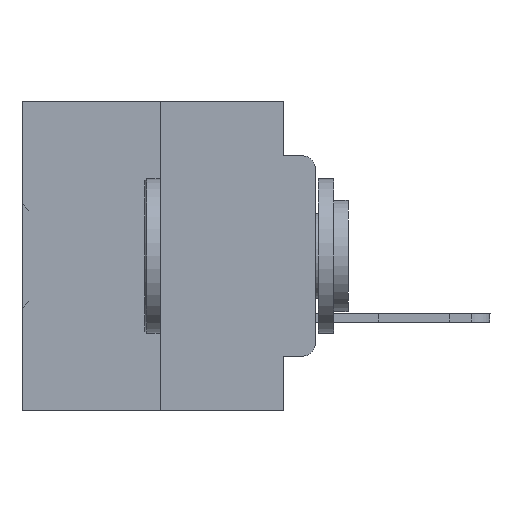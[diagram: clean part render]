
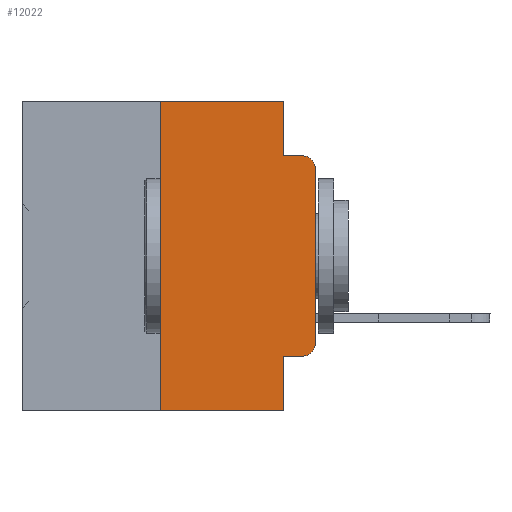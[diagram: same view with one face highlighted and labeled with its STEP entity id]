
A CAD part, left-side view. The second image highlights one B-rep face of the part: STEP entity #12022.
In plain terms, the highlighted planar face has unit normal (-1, 0, 0).
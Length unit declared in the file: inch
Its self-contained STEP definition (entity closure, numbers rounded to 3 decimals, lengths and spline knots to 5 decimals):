
#242 = CARTESIAN_POINT ( 'NONE',  ( 0., 0.051, -0.5 ) ) ;
#499 = VERTEX_POINT ( 'NONE', #16142 ) ;
#1113 = VERTEX_POINT ( 'NONE', #6329 ) ;
#1200 = CARTESIAN_POINT ( 'NONE',  ( 0., 0., 0. ) ) ;
#1485 = ORIENTED_EDGE ( 'NONE', *, *, #6885, .T. ) ;
#2350 = EDGE_LOOP ( 'NONE', ( #1485, #3402, #27702, #34656, #17338, #6366, #14215, #23502, #6802, #17267 ) ) ;
#2783 = CARTESIAN_POINT ( 'NONE',  ( 0., 0.051, 0. ) ) ;
#3402 = ORIENTED_EDGE ( 'NONE', *, *, #23648, .T. ) ;
#3685 = EDGE_CURVE ( 'NONE', #499, #12463, #12666, .T. ) ;
#3968 = AXIS2_PLACEMENT_3D ( 'NONE', #9391, #18183, #12584 ) ;
#4217 = CARTESIAN_POINT ( 'NONE',  ( 0., 0.02, -0.0885 ) ) ;
#4499 = DIRECTION ( 'NONE',  ( -1., 0., 0. ) ) ;
#6285 = EDGE_CURVE ( 'NONE', #24233, #22573, #33407, .T. ) ;
#6329 = CARTESIAN_POINT ( 'NONE',  ( 0., 0., -0.3915 ) ) ;
#6366 = ORIENTED_EDGE ( 'NONE', *, *, #29051, .F. ) ;
#6802 = ORIENTED_EDGE ( 'NONE', *, *, #15076, .T. ) ;
#6885 = EDGE_CURVE ( 'NONE', #1113, #14696, #16119, .T. ) ;
#7456 = VECTOR ( 'NONE', #12793, 39.37008 ) ;
#8163 = AXIS2_PLACEMENT_3D ( 'NONE', #16338, #4499, #36619 ) ;
#9061 = CARTESIAN_POINT ( 'NONE',  ( 0., 0.051, -0.4115 ) ) ;
#9391 = CARTESIAN_POINT ( 'NONE',  ( 0., 0.02, -0.3915 ) ) ;
#9867 = AXIS2_PLACEMENT_3D ( 'NONE', #21654, #36459, #24862 ) ;
#11653 = DIRECTION ( 'NONE',  ( 0., -1., 0. ) ) ;
#11797 = VERTEX_POINT ( 'NONE', #32631 ) ;
#12022 = ADVANCED_FACE ( 'NONE', ( #35374 ), #21527, .F. ) ;
#12463 = VERTEX_POINT ( 'NONE', #242 ) ;
#12584 = DIRECTION ( 'NONE',  ( 0., 0., -1. ) ) ;
#12666 = LINE ( 'NONE', #26035, #26336 ) ;
#12793 = DIRECTION ( 'NONE',  ( 0., 0., 1. ) ) ;
#13643 = VECTOR ( 'NONE', #28570, 39.37008 ) ;
#14215 = ORIENTED_EDGE ( 'NONE', *, *, #3685, .T. ) ;
#14696 = VERTEX_POINT ( 'NONE', #34151 ) ;
#15076 = EDGE_CURVE ( 'NONE', #20604, #37210, #22334, .T. ) ;
#15161 = CARTESIAN_POINT ( 'NONE',  ( 0., 0.051, 0. ) ) ;
#16119 = LINE ( 'NONE', #1200, #7456 ) ;
#16142 = CARTESIAN_POINT ( 'NONE',  ( 0., 0.25, -0.5 ) ) ;
#16237 = EDGE_CURVE ( 'NONE', #37210, #1113, #30061, .T. ) ;
#16338 = CARTESIAN_POINT ( 'NONE',  ( 0., 0.02, -0.1085 ) ) ;
#16698 = EDGE_CURVE ( 'NONE', #22573, #24324, #30026, .T. ) ;
#17267 = ORIENTED_EDGE ( 'NONE', *, *, #16237, .T. ) ;
#17338 = ORIENTED_EDGE ( 'NONE', *, *, #17422, .F. ) ;
#17422 = EDGE_CURVE ( 'NONE', #11797, #24233, #30847, .T. ) ;
#17732 = DIRECTION ( 'NONE',  ( 0., -1., 0. ) ) ;
#18183 = DIRECTION ( 'NONE',  ( -1., 0., 0. ) ) ;
#18979 = CARTESIAN_POINT ( 'NONE',  ( 0., 0.051, -0.0885 ) ) ;
#20604 = VERTEX_POINT ( 'NONE', #9061 ) ;
#21527 = PLANE ( 'NONE',  #9867 ) ;
#21654 = CARTESIAN_POINT ( 'NONE',  ( 0., 0.473, 0. ) ) ;
#21905 = VECTOR ( 'NONE', #30330, 39.37008 ) ;
#22334 = LINE ( 'NONE', #27272, #21905 ) ;
#22573 = VERTEX_POINT ( 'NONE', #18979 ) ;
#23502 = ORIENTED_EDGE ( 'NONE', *, *, #33842, .F. ) ;
#23648 = EDGE_CURVE ( 'NONE', #14696, #24324, #24792, .T. ) ;
#23706 = DIRECTION ( 'NONE',  ( 0., -1., 0. ) ) ;
#24146 = LINE ( 'NONE', #2783, #13643 ) ;
#24233 = VERTEX_POINT ( 'NONE', #15161 ) ;
#24324 = VERTEX_POINT ( 'NONE', #4217 ) ;
#24748 = VECTOR ( 'NONE', #26722, 39.37008 ) ;
#24792 = CIRCLE ( 'NONE', #8163, 0.02 ) ;
#24862 = DIRECTION ( 'NONE',  ( 0., 0., -1. ) ) ;
#25007 = VECTOR ( 'NONE', #11653, 39.37008 ) ;
#25928 = CARTESIAN_POINT ( 'NONE',  ( 0., 0.051, -0.0885 ) ) ;
#26035 = CARTESIAN_POINT ( 'NONE',  ( 0., 0.473, -0.5 ) ) ;
#26336 = VECTOR ( 'NONE', #17732, 39.37008 ) ;
#26722 = DIRECTION ( 'NONE',  ( 0., 0., -1. ) ) ;
#27272 = CARTESIAN_POINT ( 'NONE',  ( 0., 0.051, -0.4115 ) ) ;
#27591 = LINE ( 'NONE', #30853, #36247 ) ;
#27702 = ORIENTED_EDGE ( 'NONE', *, *, #16698, .F. ) ;
#28570 = DIRECTION ( 'NONE',  ( 0., 0., -1. ) ) ;
#29051 = EDGE_CURVE ( 'NONE', #499, #11797, #27591, .T. ) ;
#29474 = VECTOR ( 'NONE', #23706, 39.37008 ) ;
#30026 = LINE ( 'NONE', #25928, #25007 ) ;
#30061 = CIRCLE ( 'NONE', #3968, 0.02 ) ;
#30330 = DIRECTION ( 'NONE',  ( 0., -1., 0. ) ) ;
#30847 = LINE ( 'NONE', #32369, #29474 ) ;
#30853 = CARTESIAN_POINT ( 'NONE',  ( 0., 0.25, 0. ) ) ;
#31153 = CARTESIAN_POINT ( 'NONE',  ( 0., 0.02, -0.4115 ) ) ;
#32369 = CARTESIAN_POINT ( 'NONE',  ( 0., 0.473, 0. ) ) ;
#32631 = CARTESIAN_POINT ( 'NONE',  ( 0., 0.25, 0. ) ) ;
#33283 = DIRECTION ( 'NONE',  ( 0., 0., 1. ) ) ;
#33407 = LINE ( 'NONE', #35646, #24748 ) ;
#33842 = EDGE_CURVE ( 'NONE', #20604, #12463, #24146, .T. ) ;
#34151 = CARTESIAN_POINT ( 'NONE',  ( 0., 0., -0.1085 ) ) ;
#34656 = ORIENTED_EDGE ( 'NONE', *, *, #6285, .F. ) ;
#35374 = FACE_OUTER_BOUND ( 'NONE', #2350, .T. ) ;
#35646 = CARTESIAN_POINT ( 'NONE',  ( 0., 0.051, 0. ) ) ;
#36247 = VECTOR ( 'NONE', #33283, 39.37008 ) ;
#36459 = DIRECTION ( 'NONE',  ( 1., 0., 0. ) ) ;
#36619 = DIRECTION ( 'NONE',  ( 0., 0., -1. ) ) ;
#37210 = VERTEX_POINT ( 'NONE', #31153 ) ;
